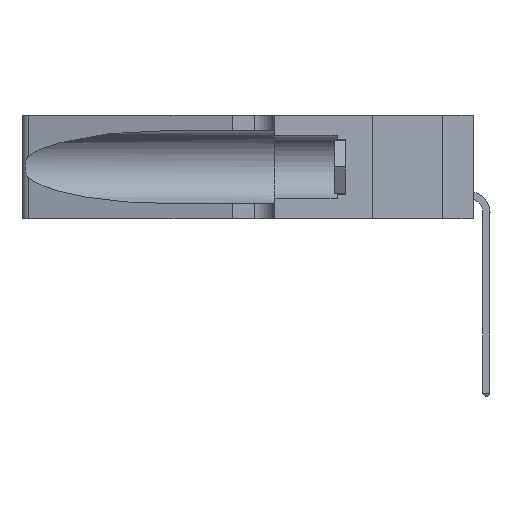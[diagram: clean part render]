
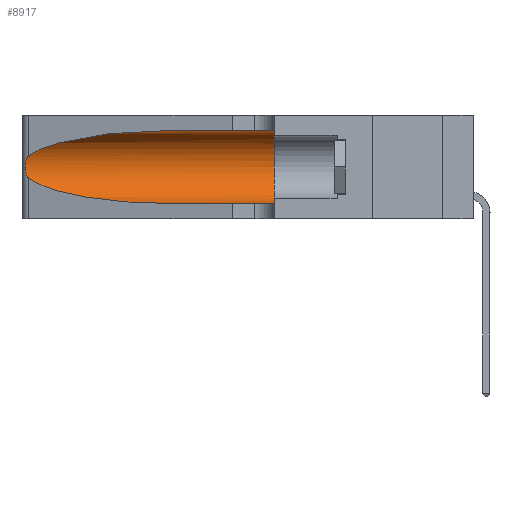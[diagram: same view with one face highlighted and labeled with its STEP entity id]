
A CAD part, left-side view. The second image highlights one B-rep face of the part: STEP entity #8917.
In plain terms, the highlighted cylindrical face has radius 3.308 mm (diameter 6.617 mm), a partial arc.
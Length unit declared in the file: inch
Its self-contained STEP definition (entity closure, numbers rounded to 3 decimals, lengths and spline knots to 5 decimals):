
#4 = VERTEX_POINT ( 'NONE', #24226 ) ;
#159 = CARTESIAN_POINT ( 'NONE',  ( 0.18966, 0.96281, 0.05475 ) ) ;
#344 = CARTESIAN_POINT ( 'NONE',  ( 0.1305, 1.61858, 0.31525 ) ) ;
#662 = AXIS2_PLACEMENT_3D ( 'NONE', #12429, #14339, #3016 ) ;
#1691 = CARTESIAN_POINT ( 'NONE',  ( 0.1305, 0.72297, 0.31525 ) ) ;
#2197 = CARTESIAN_POINT ( 'NONE',  ( 0.25555, 1.22994, 0.2215 ) ) ;
#2227 = CARTESIAN_POINT ( 'NONE',  ( 0.1305, 0.35, 0.05475 ) ) ;
#2360 = CARTESIAN_POINT ( 'NONE',  ( 0.25487, 1.22718, 0.14631 ) ) ;
#2684 = DIRECTION ( 'NONE',  ( 0., -1., 0. ) ) ;
#3016 = DIRECTION ( 'NONE',  ( 0., 0., -1. ) ) ;
#3290 = CARTESIAN_POINT ( 'NONE',  ( 0.18966, 0.96281, 0.31525 ) ) ;
#4122 = CIRCLE ( 'NONE', #19456, 0.13025 ) ;
#4182 = LINE ( 'NONE', #344, #5651 ) ;
#4335 = CARTESIAN_POINT ( 'NONE',  ( 0.26017, 1.23833, 0.17102 ) ) ;
#5174 = CARTESIAN_POINT ( 'NONE',  ( 0.2373, 1.15595, 0.28018 ) ) ;
#5434 = CARTESIAN_POINT ( 'NONE',  ( 0.25487, 1.22718, 0.22369 ) ) ;
#5587 = CARTESIAN_POINT ( 'NONE',  ( 0.25639, 1.23186, 0.15144 ) ) ;
#5651 = VECTOR ( 'NONE', #15722, 39.37008 ) ;
#5738 = CARTESIAN_POINT ( 'NONE',  ( 0.25555, 1.22993, 0.14849 ) ) ;
#7604 = CARTESIAN_POINT ( 'NONE',  ( 0.25487, 1.22718, 0.14631 ) ) ;
#8647 = CARTESIAN_POINT ( 'NONE',  ( 0.1305, 0.72297, 0.05475 ) ) ;
#8904 = CARTESIAN_POINT ( 'NONE',  ( 0.1305, 0.72297, 0.31525 ) ) ;
#8917 = ADVANCED_FACE ( 'NONE', ( #9567 ), #19113, .F. ) ;
#8936 = ORIENTED_EDGE ( 'NONE', *, *, #11567, .T. ) ;
#9567 = FACE_OUTER_BOUND ( 'NONE', #21999, .T. ) ;
#10174 = CARTESIAN_POINT ( 'NONE',  ( 0.26075, 1.23896, 0.178 ) ) ;
#10316 = VERTEX_POINT ( 'NONE', #8647 ) ;
#10443 = VERTEX_POINT ( 'NONE', #1691 ) ;
#10557 = CARTESIAN_POINT ( 'NONE',  ( 0.26018, 1.23835, 0.19895 ) ) ;
#11365 = CARTESIAN_POINT ( 'NONE',  ( 0.25487, 1.22718, 0.22369 ) ) ;
#11470 = LINE ( 'NONE', #12188, #16250 ) ;
#11567 = EDGE_CURVE ( 'NONE', #10316, #16204, #11470, .T. ) ;
#12188 = CARTESIAN_POINT ( 'NONE',  ( 0.1305, 1.61858, 0.05475 ) ) ;
#12332 = DIRECTION ( 'NONE',  ( 0., 1., 0. ) ) ;
#12429 = CARTESIAN_POINT ( 'NONE',  ( 0.1305, 1.61858, 0.185 ) ) ;
#13455 = CARTESIAN_POINT ( 'NONE',  ( 0.2373, 1.15595, 0.08982 ) ) ;
#13772 = CARTESIAN_POINT ( 'NONE',  ( 0.25639, 1.23184, 0.21858 ) ) ;
#14339 = DIRECTION ( 'NONE',  ( 0., -1., 0. ) ) ;
#14682 = ORIENTED_EDGE ( 'NONE', *, *, #18659, .T. ) ;
#15477 =( BOUNDED_CURVE ( )  B_SPLINE_CURVE ( 3, ( #2360, #13455, #159, #15530 ),
 .UNSPECIFIED., .F., .F. ) 
 B_SPLINE_CURVE_WITH_KNOTS ( ( 4, 4 ),
 ( 3.44316, 4.71239 ),
 .UNSPECIFIED. ) 
 CURVE ( )  GEOMETRIC_REPRESENTATION_ITEM ( )  RATIONAL_B_SPLINE_CURVE ( ( 1., 0.87, 0.87, 1. ) ) 
 REPRESENTATION_ITEM ( '' )  );
#15530 = CARTESIAN_POINT ( 'NONE',  ( 0.1305, 0.72297, 0.05475 ) ) ;
#15722 = DIRECTION ( 'NONE',  ( 0., -1., 0. ) ) ;
#16204 = VERTEX_POINT ( 'NONE', #2227 ) ;
#16250 = VECTOR ( 'NONE', #2684, 39.37008 ) ;
#16259 = ORIENTED_EDGE ( 'NONE', *, *, #22916, .T. ) ;
#16436 = CARTESIAN_POINT ( 'NONE',  ( 0.25856, 1.23593, 0.16098 ) ) ;
#16757 = CARTESIAN_POINT ( 'NONE',  ( 0.25787, 1.23484, 0.2124 ) ) ;
#16890 = EDGE_CURVE ( 'NONE', #10443, #4, #4182, .T. ) ;
#17315 = B_SPLINE_CURVE_WITH_KNOTS ( 'NONE', 3,
 ( #5434, #2197, #13772, #16757, #23336, #10557, #20790, #10174, #4335, #16436, #18194, #5587, #5738, #24618 ),
 .UNSPECIFIED., .F., .F.,
 ( 4, 2, 2, 2, 2, 2, 4 ),
 ( 0., 0.00027, 0.00053, 0.00107, 0.0016, 0.00187, 0.00214 ),
 .UNSPECIFIED. ) ;
#17760 =( BOUNDED_CURVE ( )  B_SPLINE_CURVE ( 3, ( #8904, #3290, #5174, #11365 ),
 .UNSPECIFIED., .F., .F. ) 
 B_SPLINE_CURVE_WITH_KNOTS ( ( 4, 4 ),
 ( 1.5708, 2.84003 ),
 .UNSPECIFIED. ) 
 CURVE ( )  GEOMETRIC_REPRESENTATION_ITEM ( )  RATIONAL_B_SPLINE_CURVE ( ( 1., 0.87, 0.87, 1. ) ) 
 REPRESENTATION_ITEM ( '' )  );
#18194 = CARTESIAN_POINT ( 'NONE',  ( 0.25789, 1.23486, 0.15765 ) ) ;
#18422 = EDGE_CURVE ( 'NONE', #23689, #23712, #17315, .T. ) ;
#18659 = EDGE_CURVE ( 'NONE', #23712, #10316, #15477, .T. ) ;
#19113 = CYLINDRICAL_SURFACE ( 'NONE', #662, 0.13025 ) ;
#19456 = AXIS2_PLACEMENT_3D ( 'NONE', #23438, #12332, #23599 ) ;
#20790 = CARTESIAN_POINT ( 'NONE',  ( 0.26075, 1.23896, 0.19203 ) ) ;
#21229 = EDGE_CURVE ( 'NONE', #4, #16204, #4122, .T. ) ;
#21703 = ORIENTED_EDGE ( 'NONE', *, *, #18422, .T. ) ;
#21774 = ORIENTED_EDGE ( 'NONE', *, *, #21229, .F. ) ;
#21999 = EDGE_LOOP ( 'NONE', ( #16259, #21703, #14682, #8936, #21774, #23445 ) ) ;
#22857 = CARTESIAN_POINT ( 'NONE',  ( 0.25487, 1.22718, 0.22369 ) ) ;
#22916 = EDGE_CURVE ( 'NONE', #10443, #23689, #17760, .T. ) ;
#23336 = CARTESIAN_POINT ( 'NONE',  ( 0.25854, 1.2359, 0.20912 ) ) ;
#23438 = CARTESIAN_POINT ( 'NONE',  ( 0.1305, 0.35, 0.185 ) ) ;
#23445 = ORIENTED_EDGE ( 'NONE', *, *, #16890, .F. ) ;
#23599 = DIRECTION ( 'NONE',  ( 0., 0., 1. ) ) ;
#23689 = VERTEX_POINT ( 'NONE', #22857 ) ;
#23712 = VERTEX_POINT ( 'NONE', #7604 ) ;
#24226 = CARTESIAN_POINT ( 'NONE',  ( 0.1305, 0.35, 0.31525 ) ) ;
#24618 = CARTESIAN_POINT ( 'NONE',  ( 0.25487, 1.22718, 0.14631 ) ) ;
